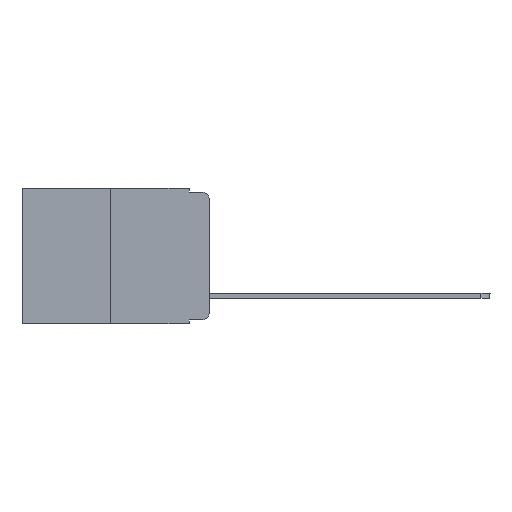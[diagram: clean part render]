
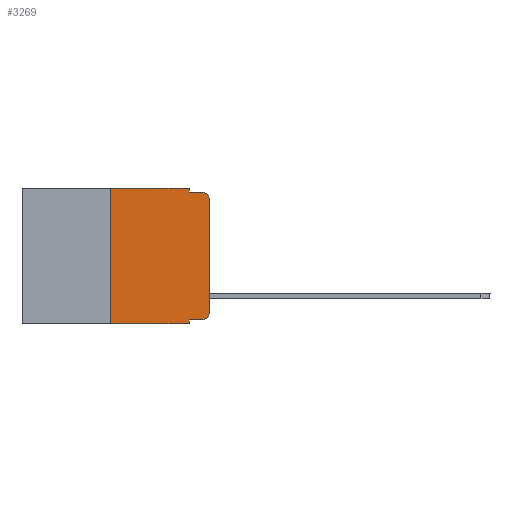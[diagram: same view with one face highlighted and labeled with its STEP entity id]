
A CAD part, left-side view. The second image highlights one B-rep face of the part: STEP entity #3269.
In plain terms, the highlighted planar face has unit normal (-1, 0, 0).
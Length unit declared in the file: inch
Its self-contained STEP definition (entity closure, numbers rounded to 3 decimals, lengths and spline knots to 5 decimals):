
#96 = VERTEX_POINT ( 'NONE', #12877 ) ;
#155 = VECTOR ( 'NONE', #13312, 39.37008 ) ;
#188 = ORIENTED_EDGE ( 'NONE', *, *, #10863, .T. ) ;
#211 = LINE ( 'NONE', #11584, #1966 ) ;
#228 = VECTOR ( 'NONE', #3525, 39.37008 ) ;
#575 = DIRECTION ( 'NONE',  ( 0., -1., 0. ) ) ;
#636 = ORIENTED_EDGE ( 'NONE', *, *, #13180, .T. ) ;
#837 = LINE ( 'NONE', #6554, #3116 ) ;
#983 = AXIS2_PLACEMENT_3D ( 'NONE', #9645, #7452, #5276 ) ;
#1364 = ORIENTED_EDGE ( 'NONE', *, *, #8203, .F. ) ;
#1373 = EDGE_CURVE ( 'NONE', #11480, #13836, #2041, .T. ) ;
#1764 = ORIENTED_EDGE ( 'NONE', *, *, #7693, .F. ) ;
#1797 = FACE_OUTER_BOUND ( 'NONE', #13965, .T. ) ;
#1855 = EDGE_CURVE ( 'NONE', #10945, #12219, #837, .T. ) ;
#1869 = PLANE ( 'NONE',  #983 ) ;
#1966 = VECTOR ( 'NONE', #13808, 39.37008 ) ;
#2041 = LINE ( 'NONE', #14360, #5684 ) ;
#2793 = CARTESIAN_POINT ( 'NONE',  ( 0., 0.473, 0. ) ) ;
#2801 = DIRECTION ( 'NONE',  ( 0., 0., -1. ) ) ;
#2825 = CIRCLE ( 'NONE', #14202, 0.02 ) ;
#2956 = LINE ( 'NONE', #2793, #9800 ) ;
#3106 = VECTOR ( 'NONE', #8468, 39.37008 ) ;
#3116 = VECTOR ( 'NONE', #5428, 39.37008 ) ;
#3269 = ADVANCED_FACE ( 'NONE', ( #1797 ), #1869, .F. ) ;
#3525 = DIRECTION ( 'NONE',  ( 0., 0., 1. ) ) ;
#3609 = ORIENTED_EDGE ( 'NONE', *, *, #3952, .T. ) ;
#3926 = LINE ( 'NONE', #13152, #3106 ) ;
#3931 = ORIENTED_EDGE ( 'NONE', *, *, #4679, .F. ) ;
#3952 = EDGE_CURVE ( 'NONE', #8897, #6316, #10860, .T. ) ;
#4328 = LINE ( 'NONE', #5357, #155 ) ;
#4679 = EDGE_CURVE ( 'NONE', #10945, #14005, #3926, .T. ) ;
#5276 = DIRECTION ( 'NONE',  ( 0., 0., -1. ) ) ;
#5357 = CARTESIAN_POINT ( 'NONE',  ( 0., 0.051, -0.01 ) ) ;
#5428 = DIRECTION ( 'NONE',  ( 0., -1., 0. ) ) ;
#5684 = VECTOR ( 'NONE', #9757, 39.37008 ) ;
#5749 = CARTESIAN_POINT ( 'NONE',  ( 0., 0.02, -0.313 ) ) ;
#5941 = CARTESIAN_POINT ( 'NONE',  ( 0., 0., -0.03 ) ) ;
#6219 = CARTESIAN_POINT ( 'NONE',  ( 0., 0.473, -0.343 ) ) ;
#6289 = CARTESIAN_POINT ( 'NONE',  ( 0., 0.051, 0. ) ) ;
#6316 = VERTEX_POINT ( 'NONE', #14241 ) ;
#6554 = CARTESIAN_POINT ( 'NONE',  ( 0., 0.051, -0.333 ) ) ;
#7076 = CARTESIAN_POINT ( 'NONE',  ( 0., 0.25, -0.343 ) ) ;
#7106 = CARTESIAN_POINT ( 'NONE',  ( 0., 0., 0. ) ) ;
#7267 = CARTESIAN_POINT ( 'NONE',  ( 0., 0.02, -0.03 ) ) ;
#7452 = DIRECTION ( 'NONE',  ( 1., 0., 0. ) ) ;
#7521 = ORIENTED_EDGE ( 'NONE', *, *, #1855, .T. ) ;
#7693 = EDGE_CURVE ( 'NONE', #10893, #96, #211, .T. ) ;
#8203 = EDGE_CURVE ( 'NONE', #13836, #10893, #2956, .T. ) ;
#8214 = CARTESIAN_POINT ( 'NONE',  ( 0., 0.051, -0.343 ) ) ;
#8451 = CARTESIAN_POINT ( 'NONE',  ( 0., 0.25, 0. ) ) ;
#8468 = DIRECTION ( 'NONE',  ( 0., 0., -1. ) ) ;
#8668 = LINE ( 'NONE', #6219, #10838 ) ;
#8835 = CARTESIAN_POINT ( 'NONE',  ( 0., 0.02, -0.333 ) ) ;
#8897 = VERTEX_POINT ( 'NONE', #5941 ) ;
#9220 = DIRECTION ( 'NONE',  ( 0., 0., -1. ) ) ;
#9615 = DIRECTION ( 'NONE',  ( 0., -1., 0. ) ) ;
#9645 = CARTESIAN_POINT ( 'NONE',  ( 0., 0.473, 0. ) ) ;
#9757 = DIRECTION ( 'NONE',  ( 0., 0., 1. ) ) ;
#9800 = VECTOR ( 'NONE', #9615, 39.37008 ) ;
#10604 = EDGE_CURVE ( 'NONE', #96, #6316, #4328, .T. ) ;
#10838 = VECTOR ( 'NONE', #575, 39.37008 ) ;
#10860 = CIRCLE ( 'NONE', #13930, 0.02 ) ;
#10863 = EDGE_CURVE ( 'NONE', #11480, #14005, #8668, .T. ) ;
#10893 = VERTEX_POINT ( 'NONE', #6289 ) ;
#10945 = VERTEX_POINT ( 'NONE', #14381 ) ;
#10989 = CARTESIAN_POINT ( 'NONE',  ( 0., 0., -0.313 ) ) ;
#11108 = ORIENTED_EDGE ( 'NONE', *, *, #1373, .F. ) ;
#11480 = VERTEX_POINT ( 'NONE', #7076 ) ;
#11584 = CARTESIAN_POINT ( 'NONE',  ( 0., 0.051, 0. ) ) ;
#11796 = DIRECTION ( 'NONE',  ( -1., 0., 0. ) ) ;
#12219 = VERTEX_POINT ( 'NONE', #8835 ) ;
#12877 = CARTESIAN_POINT ( 'NONE',  ( 0., 0.051, -0.01 ) ) ;
#13002 = ORIENTED_EDGE ( 'NONE', *, *, #10604, .F. ) ;
#13152 = CARTESIAN_POINT ( 'NONE',  ( 0., 0.051, 0. ) ) ;
#13180 = EDGE_CURVE ( 'NONE', #12219, #13823, #2825, .T. ) ;
#13312 = DIRECTION ( 'NONE',  ( 0., -1., 0. ) ) ;
#13698 = LINE ( 'NONE', #7106, #228 ) ;
#13808 = DIRECTION ( 'NONE',  ( 0., 0., -1. ) ) ;
#13823 = VERTEX_POINT ( 'NONE', #10989 ) ;
#13831 = DIRECTION ( 'NONE',  ( -1., 0., 0. ) ) ;
#13836 = VERTEX_POINT ( 'NONE', #8451 ) ;
#13930 = AXIS2_PLACEMENT_3D ( 'NONE', #7267, #11796, #2801 ) ;
#13965 = EDGE_LOOP ( 'NONE', ( #14040, #3609, #13002, #1764, #1364, #11108, #188, #3931, #7521, #636 ) ) ;
#14005 = VERTEX_POINT ( 'NONE', #8214 ) ;
#14040 = ORIENTED_EDGE ( 'NONE', *, *, #14061, .T. ) ;
#14061 = EDGE_CURVE ( 'NONE', #13823, #8897, #13698, .T. ) ;
#14202 = AXIS2_PLACEMENT_3D ( 'NONE', #5749, #13831, #9220 ) ;
#14241 = CARTESIAN_POINT ( 'NONE',  ( 0., 0.02, -0.01 ) ) ;
#14360 = CARTESIAN_POINT ( 'NONE',  ( 0., 0.25, 0. ) ) ;
#14381 = CARTESIAN_POINT ( 'NONE',  ( 0., 0.051, -0.333 ) ) ;
